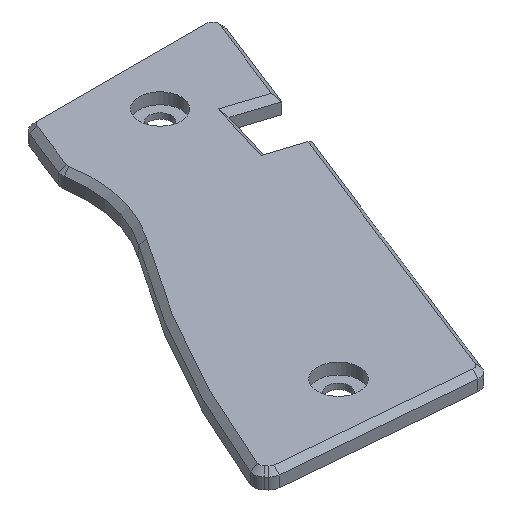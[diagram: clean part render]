
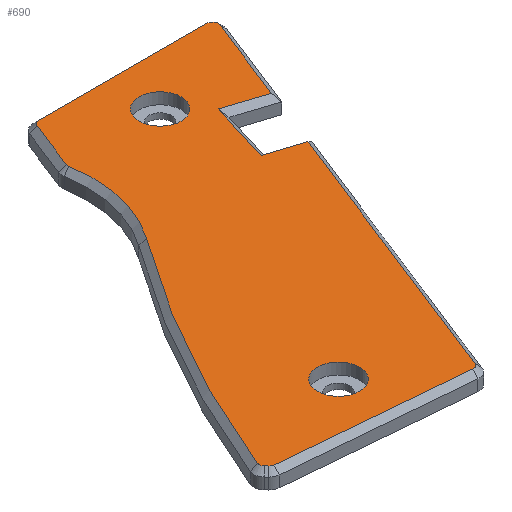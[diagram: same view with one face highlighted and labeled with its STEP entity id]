
A CAD part, isometric view. The second image highlights one B-rep face of the part: STEP entity #690.
In plain terms, the highlighted planar face has unit normal (0, 0, 1).
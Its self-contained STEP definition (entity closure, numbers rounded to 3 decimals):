
#15=FACE_BOUND('',#143,.T.);
#16=FACE_BOUND('',#144,.T.);
#34=CIRCLE('',#722,1.);
#36=CIRCLE('',#726,1.);
#38=CIRCLE('',#730,1.);
#40=CIRCLE('',#733,23.992);
#43=CIRCLE('',#738,204.75);
#44=CIRCLE('',#740,1.);
#46=CIRCLE('',#744,1.);
#48=CIRCLE('',#748,1.);
#56=CIRCLE('',#769,3.75);
#57=CIRCLE('',#770,3.75);
#100=FACE_OUTER_BOUND('',#142,.T.);
#142=EDGE_LOOP('',(#552,#553,#554,#555,#556,#557,#558,#559,#560,#561,#562,
#563,#564,#565,#566,#567,#568));
#143=EDGE_LOOP('',(#569));
#144=EDGE_LOOP('',(#570));
#166=LINE('',#1016,#230);
#170=LINE('',#1028,#234);
#174=LINE('',#1040,#238);
#178=LINE('',#1067,#242);
#183=LINE('',#1085,#247);
#187=LINE('',#1097,#251);
#190=LINE('',#1107,#254);
#194=LINE('',#1115,#258);
#196=LINE('',#1118,#260);
#230=VECTOR('',#800,10.);
#234=VECTOR('',#812,10.);
#238=VECTOR('',#824,10.);
#242=VECTOR('',#842,10.);
#247=VECTOR('',#861,10.);
#251=VECTOR('',#873,10.);
#254=VECTOR('',#884,10.);
#258=VECTOR('',#890,10.);
#260=VECTOR('',#894,10.);
#294=VERTEX_POINT('',#1013);
#295=VERTEX_POINT('',#1015);
#297=VERTEX_POINT('',#1020);
#299=VERTEX_POINT('',#1026);
#301=VERTEX_POINT('',#1032);
#303=VERTEX_POINT('',#1038);
#305=VERTEX_POINT('',#1044);
#307=VERTEX_POINT('',#1050);
#309=VERTEX_POINT('',#1066);
#311=VERTEX_POINT('',#1072);
#313=VERTEX_POINT('',#1077);
#315=VERTEX_POINT('',#1083);
#317=VERTEX_POINT('',#1089);
#319=VERTEX_POINT('',#1095);
#321=VERTEX_POINT('',#1101);
#322=VERTEX_POINT('',#1106);
#325=VERTEX_POINT('',#1114);
#336=VERTEX_POINT('',#1159);
#337=VERTEX_POINT('',#1161);
#353=EDGE_CURVE('',#294,#295,#166,.T.);
#356=EDGE_CURVE('',#297,#294,#34,.T.);
#359=EDGE_CURVE('',#299,#297,#170,.T.);
#362=EDGE_CURVE('',#301,#299,#36,.T.);
#365=EDGE_CURVE('',#303,#301,#174,.T.);
#368=EDGE_CURVE('',#305,#303,#38,.T.);
#371=EDGE_CURVE('',#307,#305,#40,.T.);
#374=EDGE_CURVE('',#295,#309,#178,.T.);
#378=EDGE_CURVE('',#311,#307,#43,.T.);
#380=EDGE_CURVE('',#313,#311,#44,.T.);
#383=EDGE_CURVE('',#315,#313,#183,.T.);
#386=EDGE_CURVE('',#317,#315,#46,.T.);
#389=EDGE_CURVE('',#319,#317,#187,.T.);
#392=EDGE_CURVE('',#321,#319,#48,.T.);
#394=EDGE_CURVE('',#322,#321,#190,.T.);
#398=EDGE_CURVE('',#309,#325,#194,.T.);
#400=EDGE_CURVE('',#325,#322,#196,.T.);
#421=EDGE_CURVE('',#336,#336,#56,.F.);
#422=EDGE_CURVE('',#337,#337,#57,.F.);
#552=ORIENTED_EDGE('',*,*,#353,.F.);
#553=ORIENTED_EDGE('',*,*,#356,.F.);
#554=ORIENTED_EDGE('',*,*,#359,.F.);
#555=ORIENTED_EDGE('',*,*,#362,.F.);
#556=ORIENTED_EDGE('',*,*,#365,.F.);
#557=ORIENTED_EDGE('',*,*,#368,.F.);
#558=ORIENTED_EDGE('',*,*,#371,.F.);
#559=ORIENTED_EDGE('',*,*,#378,.F.);
#560=ORIENTED_EDGE('',*,*,#380,.F.);
#561=ORIENTED_EDGE('',*,*,#383,.F.);
#562=ORIENTED_EDGE('',*,*,#386,.F.);
#563=ORIENTED_EDGE('',*,*,#389,.F.);
#564=ORIENTED_EDGE('',*,*,#392,.F.);
#565=ORIENTED_EDGE('',*,*,#394,.F.);
#566=ORIENTED_EDGE('',*,*,#400,.F.);
#567=ORIENTED_EDGE('',*,*,#398,.F.);
#568=ORIENTED_EDGE('',*,*,#374,.F.);
#569=ORIENTED_EDGE('',*,*,#421,.T.);
#570=ORIENTED_EDGE('',*,*,#422,.T.);
#654=PLANE('',#768);
#690=ADVANCED_FACE('',(#100,#15,#16),#654,.F.);
#722=AXIS2_PLACEMENT_3D('',#1022,#805,#806);
#726=AXIS2_PLACEMENT_3D('',#1034,#817,#818);
#730=AXIS2_PLACEMENT_3D('',#1046,#829,#830);
#733=AXIS2_PLACEMENT_3D('',#1061,#835,#836);
#738=AXIS2_PLACEMENT_3D('',#1074,#849,#850);
#740=AXIS2_PLACEMENT_3D('',#1079,#854,#855);
#744=AXIS2_PLACEMENT_3D('',#1091,#866,#867);
#748=AXIS2_PLACEMENT_3D('',#1103,#878,#879);
#768=AXIS2_PLACEMENT_3D('',#1158,#939,#940);
#769=AXIS2_PLACEMENT_3D('',#1160,#941,#942);
#770=AXIS2_PLACEMENT_3D('',#1162,#943,#944);
#800=DIRECTION('',(-0.367,-0.93,0.));
#805=DIRECTION('center_axis',(0.,0.,-1.));
#806=DIRECTION('ref_axis',(0.827,0.563,0.));
#812=DIRECTION('',(1.,0.,0.));
#817=DIRECTION('center_axis',(0.,0.,-1.));
#818=DIRECTION('ref_axis',(-0.563,0.827,0.));
#824=DIRECTION('',(0.367,0.93,0.));
#829=DIRECTION('center_axis',(0.,0.,-1.));
#830=DIRECTION('ref_axis',(-0.995,0.103,0.));
#835=DIRECTION('center_axis',(0.,0.,1.));
#836=DIRECTION('ref_axis',(0.98,0.2,0.));
#842=DIRECTION('',(-0.951,0.31,0.));
#849=DIRECTION('center_axis',(0.,0.,-1.));
#850=DIRECTION('ref_axis',(-0.93,0.367,0.));
#854=DIRECTION('center_axis',(0.,0.,-1.));
#855=DIRECTION('ref_axis',(-0.982,-0.191,0.));
#861=DIRECTION('',(-0.694,0.72,0.));
#866=DIRECTION('center_axis',(0.,0.,-1.));
#867=DIRECTION('ref_axis',(-0.432,-0.902,0.));
#873=DIRECTION('',(-0.996,0.089,0.));
#878=DIRECTION('center_axis',(0.,0.,-1.));
#879=DIRECTION('ref_axis',(0.525,-0.851,0.));
#884=DIRECTION('',(-0.367,-0.93,0.));
#890=DIRECTION('',(-0.292,-0.956,0.));
#894=DIRECTION('',(0.951,-0.31,0.));
#939=DIRECTION('center_axis',(0.,0.,-1.));
#940=DIRECTION('ref_axis',(1.,0.,0.));
#941=DIRECTION('center_axis',(0.,0.,1.));
#942=DIRECTION('ref_axis',(-1.,0.,0.));
#943=DIRECTION('center_axis',(0.,0.,1.));
#944=DIRECTION('ref_axis',(-1.,0.,0.));
#1013=CARTESIAN_POINT('',(61.469,-15.43,16.9));
#1015=CARTESIAN_POINT('',(55.486,-30.62,16.9));
#1016=CARTESIAN_POINT('',(54.34,-33.53,16.9));
#1020=CARTESIAN_POINT('',(60.539,-14.063,16.9));
#1022=CARTESIAN_POINT('Origin',(60.539,-15.063,16.9));
#1026=CARTESIAN_POINT('',(30.503,-14.063,16.9));
#1028=CARTESIAN_POINT('',(34.438,-14.063,16.9));
#1032=CARTESIAN_POINT('',(29.573,-14.697,16.9));
#1034=CARTESIAN_POINT('Origin',(30.503,-15.063,16.9));
#1038=CARTESIAN_POINT('',(26.197,-23.266,16.9));
#1040=CARTESIAN_POINT('',(22.773,-31.96,16.9));
#1044=CARTESIAN_POINT('',(26.142,-23.8,16.9));
#1046=CARTESIAN_POINT('Origin',(27.128,-23.632,16.9));
#1050=CARTESIAN_POINT('',(21.901,-41.92,16.9));
#1061=CARTESIAN_POINT('Origin',(2.489,-27.821,16.9));
#1066=CARTESIAN_POINT('',(48.317,-28.281,16.9));
#1067=CARTESIAN_POINT('',(50.784,-29.086,16.9));
#1072=CARTESIAN_POINT('',(-2.919,-86.537,16.9));
#1074=CARTESIAN_POINT('Origin',(187.022,-162.989,16.9));
#1077=CARTESIAN_POINT('',(-2.712,-87.604,16.9));
#1079=CARTESIAN_POINT('Origin',(-1.992,-86.91,16.9));
#1083=CARTESIAN_POINT('',(-2.338,-87.992,16.9));
#1085=CARTESIAN_POINT('',(-2.493,-87.831,16.9));
#1089=CARTESIAN_POINT('',(-1.707,-88.294,16.9));
#1091=CARTESIAN_POINT('Origin',(-1.618,-87.298,16.9));
#1095=CARTESIAN_POINT('',(30.851,-91.202,16.9));
#1097=CARTESIAN_POINT('',(32.675,-91.364,16.9));
#1101=CARTESIAN_POINT('',(31.87,-90.572,16.9));
#1103=CARTESIAN_POINT('Origin',(30.94,-90.206,16.9));
#1106=CARTESIAN_POINT('',(51.257,-41.355,16.9));
#1107=CARTESIAN_POINT('',(54.34,-33.53,16.9));
#1114=CARTESIAN_POINT('',(44.956,-39.299,16.9));
#1115=CARTESIAN_POINT('',(44.972,-39.244,16.9));
#1118=CARTESIAN_POINT('',(43.752,-38.906,16.9));
#1158=CARTESIAN_POINT('Origin',(38.373,-48.148,16.9));
#1159=CARTESIAN_POINT('',(21.042,-80.791,16.9));
#1160=CARTESIAN_POINT('Origin',(17.292,-80.791,16.9));
#1161=CARTESIAN_POINT('',(46.882,-23.118,16.9));
#1162=CARTESIAN_POINT('Origin',(43.132,-23.118,16.9));
